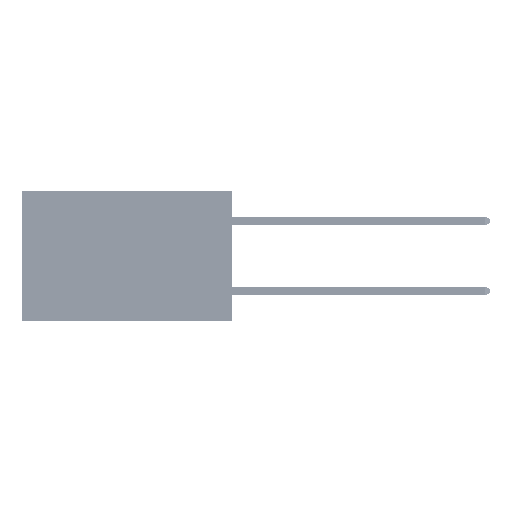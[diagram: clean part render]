
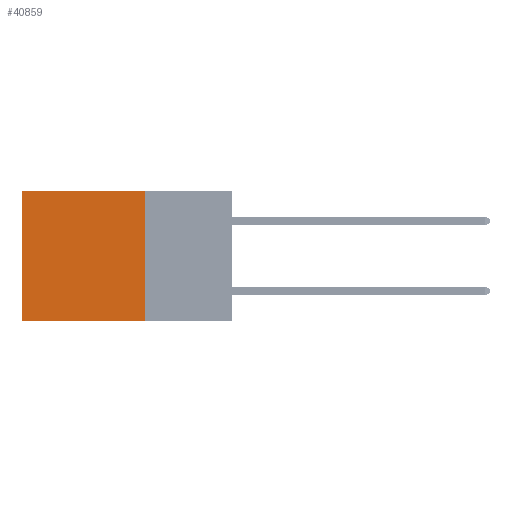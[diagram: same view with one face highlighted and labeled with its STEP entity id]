
A CAD part, left-side view. The second image highlights one B-rep face of the part: STEP entity #40859.
In plain terms, the highlighted planar face has unit normal (-1, 0, 0).
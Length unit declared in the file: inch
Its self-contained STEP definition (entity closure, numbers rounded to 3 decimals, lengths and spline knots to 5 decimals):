
#255 = ORIENTED_EDGE ( 'NONE', *, *, #11048, .T. ) ;
#5910 = VECTOR ( 'NONE', #48126, 39.37008 ) ;
#6712 = CARTESIAN_POINT ( 'NONE',  ( 0.2875, 0.25, -0.37 ) ) ;
#8787 = DIRECTION ( 'NONE',  ( 0., 0., -1. ) ) ;
#11048 = EDGE_CURVE ( 'NONE', #14211, #22324, #17991, .T. ) ;
#11691 = AXIS2_PLACEMENT_3D ( 'NONE', #24819, #28614, #8787 ) ;
#11900 = ORIENTED_EDGE ( 'NONE', *, *, #19812, .T. ) ;
#14211 = VERTEX_POINT ( 'NONE', #22991 ) ;
#15483 = VECTOR ( 'NONE', #49531, 39.37008 ) ;
#15802 = CARTESIAN_POINT ( 'NONE',  ( 0.2875, 0.6, -0.37 ) ) ;
#15953 = CARTESIAN_POINT ( 'NONE',  ( 0.2875, 0.25, 0. ) ) ;
#17991 = LINE ( 'NONE', #44496, #15483 ) ;
#18537 = CARTESIAN_POINT ( 'NONE',  ( 0.2875, 0.25, 0. ) ) ;
#19699 = LINE ( 'NONE', #43791, #5910 ) ;
#19812 = EDGE_CURVE ( 'NONE', #24889, #14211, #41101, .T. ) ;
#22030 = DIRECTION ( 'NONE',  ( 0., 1., 0. ) ) ;
#22324 = VERTEX_POINT ( 'NONE', #15802 ) ;
#22991 = CARTESIAN_POINT ( 'NONE',  ( 0.2875, 0.6, 0. ) ) ;
#24426 = LINE ( 'NONE', #15953, #39319 ) ;
#24819 = CARTESIAN_POINT ( 'NONE',  ( 0.2875, 0.25, 0. ) ) ;
#24889 = VERTEX_POINT ( 'NONE', #30787 ) ;
#25227 = EDGE_LOOP ( 'NONE', ( #255, #50208, #39031, #11900 ) ) ;
#27542 = FACE_OUTER_BOUND ( 'NONE', #25227, .T. ) ;
#28614 = DIRECTION ( 'NONE',  ( 1., 0., 0. ) ) ;
#30787 = CARTESIAN_POINT ( 'NONE',  ( 0.2875, 0.25, 0. ) ) ;
#33633 = VECTOR ( 'NONE', #22030, 39.37008 ) ;
#35727 = DIRECTION ( 'NONE',  ( 0., 0., -1. ) ) ;
#36952 = PLANE ( 'NONE',  #11691 ) ;
#38206 = EDGE_CURVE ( 'NONE', #44629, #22324, #19699, .T. ) ;
#39031 = ORIENTED_EDGE ( 'NONE', *, *, #49120, .F. ) ;
#39319 = VECTOR ( 'NONE', #35727, 39.37008 ) ;
#40859 = ADVANCED_FACE ( 'NONE', ( #27542 ), #36952, .F. ) ;
#41101 = LINE ( 'NONE', #18537, #33633 ) ;
#43791 = CARTESIAN_POINT ( 'NONE',  ( 0.2875, 0.25, -0.37 ) ) ;
#44496 = CARTESIAN_POINT ( 'NONE',  ( 0.2875, 0.6, 0. ) ) ;
#44629 = VERTEX_POINT ( 'NONE', #6712 ) ;
#48126 = DIRECTION ( 'NONE',  ( 0., 1., 0. ) ) ;
#49120 = EDGE_CURVE ( 'NONE', #24889, #44629, #24426, .T. ) ;
#49531 = DIRECTION ( 'NONE',  ( 0., 0., -1. ) ) ;
#50208 = ORIENTED_EDGE ( 'NONE', *, *, #38206, .F. ) ;
